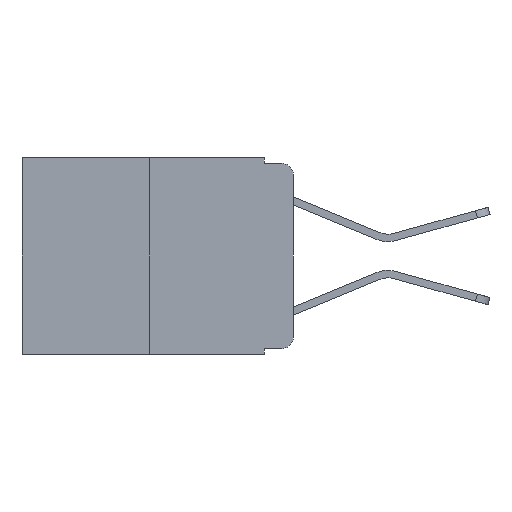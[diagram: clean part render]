
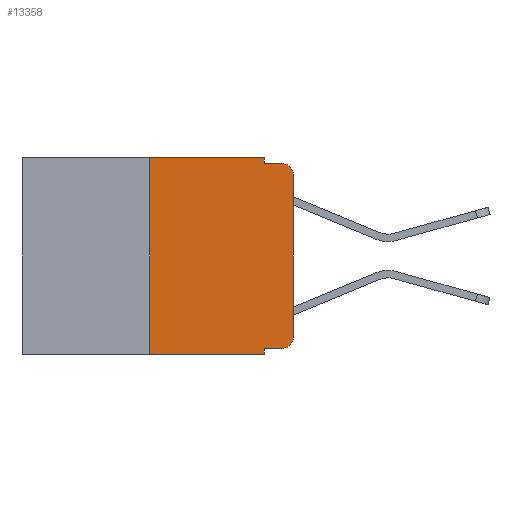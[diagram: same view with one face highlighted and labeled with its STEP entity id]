
A CAD part, left-side view. The second image highlights one B-rep face of the part: STEP entity #13358.
In plain terms, the highlighted planar face has unit normal (-1, 0, 0).
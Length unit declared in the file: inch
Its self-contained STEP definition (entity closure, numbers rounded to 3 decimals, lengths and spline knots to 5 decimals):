
#50 = EDGE_CURVE ( 'NONE', #15914, #9243, #758, .T. ) ;
#396 = CARTESIAN_POINT ( 'NONE',  ( 0., 0.051, 0. ) ) ;
#461 = CARTESIAN_POINT ( 'NONE',  ( 0., 0.051, 0. ) ) ;
#521 = VECTOR ( 'NONE', #9626, 39.37008 ) ;
#564 = DIRECTION ( 'NONE',  ( 1., 0., 0. ) ) ;
#634 = CARTESIAN_POINT ( 'NONE',  ( 0., 0.25, -0.343 ) ) ;
#669 = DIRECTION ( 'NONE',  ( 0., 0., 1. ) ) ;
#701 = ORIENTED_EDGE ( 'NONE', *, *, #3710, .F. ) ;
#758 = LINE ( 'NONE', #7518, #5597 ) ;
#858 = ORIENTED_EDGE ( 'NONE', *, *, #50, .T. ) ;
#2734 = CARTESIAN_POINT ( 'NONE',  ( 0., 0.25, 0. ) ) ;
#3103 = LINE ( 'NONE', #9851, #6103 ) ;
#3307 = FACE_OUTER_BOUND ( 'NONE', #5846, .T. ) ;
#3395 = CARTESIAN_POINT ( 'NONE',  ( 0., 0.02, -0.01 ) ) ;
#3710 = EDGE_CURVE ( 'NONE', #12197, #10051, #16144, .T. ) ;
#3732 = ORIENTED_EDGE ( 'NONE', *, *, #6029, .T. ) ;
#3833 = CARTESIAN_POINT ( 'NONE',  ( 0., 0.051, 0. ) ) ;
#3858 = CARTESIAN_POINT ( 'NONE',  ( 0., 0.051, -0.333 ) ) ;
#3919 = LINE ( 'NONE', #3833, #8060 ) ;
#3943 = DIRECTION ( 'NONE',  ( 0., -1., 0. ) ) ;
#4079 = CARTESIAN_POINT ( 'NONE',  ( 0., 0.051, -0.01 ) ) ;
#4441 = ORIENTED_EDGE ( 'NONE', *, *, #17184, .T. ) ;
#4714 = AXIS2_PLACEMENT_3D ( 'NONE', #15891, #9327, #8019 ) ;
#4742 = CARTESIAN_POINT ( 'NONE',  ( 0., 0.051, -0.343 ) ) ;
#4941 = VECTOR ( 'NONE', #3943, 39.37008 ) ;
#5078 = VERTEX_POINT ( 'NONE', #9666 ) ;
#5201 = LINE ( 'NONE', #3858, #4941 ) ;
#5315 = ORIENTED_EDGE ( 'NONE', *, *, #14820, .F. ) ;
#5342 = VECTOR ( 'NONE', #16416, 39.37008 ) ;
#5597 = VECTOR ( 'NONE', #669, 39.37008 ) ;
#5611 = LINE ( 'NONE', #461, #16848 ) ;
#5644 = ORIENTED_EDGE ( 'NONE', *, *, #7408, .F. ) ;
#5846 = EDGE_LOOP ( 'NONE', ( #858, #11573, #701, #5315, #15668, #5644, #3732, #6581, #10758, #4441 ) ) ;
#6029 = EDGE_CURVE ( 'NONE', #15791, #10016, #13706, .T. ) ;
#6103 = VECTOR ( 'NONE', #9667, 39.37008 ) ;
#6581 = ORIENTED_EDGE ( 'NONE', *, *, #15656, .F. ) ;
#6618 = CARTESIAN_POINT ( 'NONE',  ( 0., 0.473, -0.343 ) ) ;
#7408 = EDGE_CURVE ( 'NONE', #15791, #10756, #15266, .T. ) ;
#7518 = CARTESIAN_POINT ( 'NONE',  ( 0., 0., 0. ) ) ;
#7522 = CIRCLE ( 'NONE', #17431, 0.02 ) ;
#7740 = AXIS2_PLACEMENT_3D ( 'NONE', #14047, #564, #9975 ) ;
#8019 = DIRECTION ( 'NONE',  ( 0., 0., -1. ) ) ;
#8060 = VECTOR ( 'NONE', #15906, 39.37008 ) ;
#8699 = CARTESIAN_POINT ( 'NONE',  ( 0., 0., -0.03 ) ) ;
#9243 = VERTEX_POINT ( 'NONE', #8699 ) ;
#9327 = DIRECTION ( 'NONE',  ( -1., 0., 0. ) ) ;
#9478 = VERTEX_POINT ( 'NONE', #17281 ) ;
#9626 = DIRECTION ( 'NONE',  ( 0., -1., 0. ) ) ;
#9666 = CARTESIAN_POINT ( 'NONE',  ( 0., 0.051, -0.333 ) ) ;
#9667 = DIRECTION ( 'NONE',  ( 0., -1., 0. ) ) ;
#9685 = DIRECTION ( 'NONE',  ( 0., 0., -1. ) ) ;
#9851 = CARTESIAN_POINT ( 'NONE',  ( 0., 0.473, 0. ) ) ;
#9975 = DIRECTION ( 'NONE',  ( 0., 0., -1. ) ) ;
#10016 = VERTEX_POINT ( 'NONE', #4742 ) ;
#10051 = VERTEX_POINT ( 'NONE', #3395 ) ;
#10671 = CIRCLE ( 'NONE', #4714, 0.02 ) ;
#10749 = CARTESIAN_POINT ( 'NONE',  ( 0., 0.02, -0.03 ) ) ;
#10756 = VERTEX_POINT ( 'NONE', #2734 ) ;
#10758 = ORIENTED_EDGE ( 'NONE', *, *, #15117, .T. ) ;
#10835 = DIRECTION ( 'NONE',  ( 0., -1., 0. ) ) ;
#10939 = CARTESIAN_POINT ( 'NONE',  ( 0., 0.25, 0. ) ) ;
#11573 = ORIENTED_EDGE ( 'NONE', *, *, #15990, .T. ) ;
#12155 = DIRECTION ( 'NONE',  ( -1., 0., 0. ) ) ;
#12197 = VERTEX_POINT ( 'NONE', #4079 ) ;
#12772 = CARTESIAN_POINT ( 'NONE',  ( 0., 0., -0.313 ) ) ;
#12878 = PLANE ( 'NONE',  #7740 ) ;
#13358 = ADVANCED_FACE ( 'NONE', ( #3307 ), #12878, .F. ) ;
#13706 = LINE ( 'NONE', #6618, #521 ) ;
#14047 = CARTESIAN_POINT ( 'NONE',  ( 0., 0.473, 0. ) ) ;
#14820 = EDGE_CURVE ( 'NONE', #15281, #12197, #3919, .T. ) ;
#15117 = EDGE_CURVE ( 'NONE', #5078, #9478, #5201, .T. ) ;
#15266 = LINE ( 'NONE', #10939, #5342 ) ;
#15281 = VERTEX_POINT ( 'NONE', #396 ) ;
#15656 = EDGE_CURVE ( 'NONE', #5078, #10016, #5611, .T. ) ;
#15668 = ORIENTED_EDGE ( 'NONE', *, *, #16198, .F. ) ;
#15791 = VERTEX_POINT ( 'NONE', #634 ) ;
#15891 = CARTESIAN_POINT ( 'NONE',  ( 0., 0.02, -0.313 ) ) ;
#15906 = DIRECTION ( 'NONE',  ( 0., 0., -1. ) ) ;
#15914 = VERTEX_POINT ( 'NONE', #12772 ) ;
#15990 = EDGE_CURVE ( 'NONE', #9243, #10051, #7522, .T. ) ;
#16144 = LINE ( 'NONE', #16319, #17364 ) ;
#16149 = DIRECTION ( 'NONE',  ( 0., 0., -1. ) ) ;
#16198 = EDGE_CURVE ( 'NONE', #10756, #15281, #3103, .T. ) ;
#16319 = CARTESIAN_POINT ( 'NONE',  ( 0., 0.051, -0.01 ) ) ;
#16416 = DIRECTION ( 'NONE',  ( 0., 0., 1. ) ) ;
#16848 = VECTOR ( 'NONE', #9685, 39.37008 ) ;
#17184 = EDGE_CURVE ( 'NONE', #9478, #15914, #10671, .T. ) ;
#17281 = CARTESIAN_POINT ( 'NONE',  ( 0., 0.02, -0.333 ) ) ;
#17364 = VECTOR ( 'NONE', #10835, 39.37008 ) ;
#17431 = AXIS2_PLACEMENT_3D ( 'NONE', #10749, #12155, #16149 ) ;
